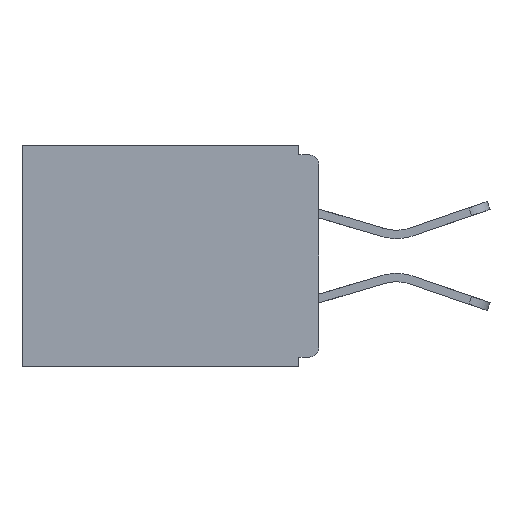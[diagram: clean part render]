
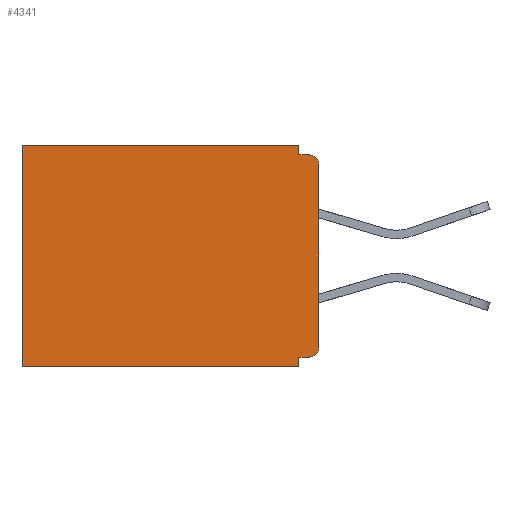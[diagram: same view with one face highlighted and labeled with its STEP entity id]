
A CAD part, left-side view. The second image highlights one B-rep face of the part: STEP entity #4341.
In plain terms, the highlighted planar face has unit normal (-1, 0, 0).
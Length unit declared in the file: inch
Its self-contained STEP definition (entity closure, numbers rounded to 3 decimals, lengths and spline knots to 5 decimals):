
#264 = VECTOR ( 'NONE', #6462, 39.37008 ) ;
#429 = LINE ( 'NONE', #3841, #842 ) ;
#657 = VECTOR ( 'NONE', #9580, 39.37008 ) ;
#702 = VECTOR ( 'NONE', #5959, 39.37008 ) ;
#765 = EDGE_CURVE ( 'NONE', #10484, #6599, #7056, .T. ) ;
#837 = EDGE_CURVE ( 'NONE', #10484, #2158, #3985, .T. ) ;
#842 = VECTOR ( 'NONE', #13046, 39.37008 ) ;
#1047 = CARTESIAN_POINT ( 'NONE',  ( 0.298, 0., -0.03 ) ) ;
#1114 = LINE ( 'NONE', #1964, #702 ) ;
#1277 = VERTEX_POINT ( 'NONE', #11123 ) ;
#1627 = EDGE_CURVE ( 'NONE', #6599, #11032, #429, .T. ) ;
#1770 = EDGE_LOOP ( 'NONE', ( #12987, #15090, #11916, #7099, #12322, #15769, #7024, #5704, #8337, #3221 ) ) ;
#1964 = CARTESIAN_POINT ( 'NONE',  ( 0.298, 0., 0. ) ) ;
#2158 = VERTEX_POINT ( 'NONE', #2825 ) ;
#2263 = DIRECTION ( 'NONE',  ( -1., 0., 0. ) ) ;
#2493 = CARTESIAN_POINT ( 'NONE',  ( 0.298, 0., -0.343 ) ) ;
#2712 = LINE ( 'NONE', #16042, #12008 ) ;
#2825 = CARTESIAN_POINT ( 'NONE',  ( 0.298, 0., -0.313 ) ) ;
#3004 = EDGE_CURVE ( 'NONE', #9972, #15395, #13359, .T. ) ;
#3078 = LINE ( 'NONE', #15502, #10525 ) ;
#3161 = CARTESIAN_POINT ( 'NONE',  ( 0.298, 0., -0.015 ) ) ;
#3221 = ORIENTED_EDGE ( 'NONE', *, *, #5200, .F. ) ;
#3610 = CARTESIAN_POINT ( 'NONE',  ( 0.298, 0.015, -0.328 ) ) ;
#3698 = DIRECTION ( 'NONE',  ( -1., 0., 0. ) ) ;
#3841 = CARTESIAN_POINT ( 'NONE',  ( 0.298, 0.031, -0.343 ) ) ;
#3985 = CIRCLE ( 'NONE', #14149, 0.015 ) ;
#4000 = DIRECTION ( 'NONE',  ( 0., 0., -1. ) ) ;
#4341 = ADVANCED_FACE ( 'NONE', ( #10231 ), #12079, .F. ) ;
#4699 = DIRECTION ( 'NONE',  ( 0., 1., 0. ) ) ;
#4863 = AXIS2_PLACEMENT_3D ( 'NONE', #5848, #9821, #5898 ) ;
#5200 = EDGE_CURVE ( 'NONE', #9972, #2158, #1114, .T. ) ;
#5704 = ORIENTED_EDGE ( 'NONE', *, *, #765, .F. ) ;
#5848 = CARTESIAN_POINT ( 'NONE',  ( 0.298, 0., 0. ) ) ;
#5898 = DIRECTION ( 'NONE',  ( 0., 0., -1. ) ) ;
#5959 = DIRECTION ( 'NONE',  ( 0., 0., -1. ) ) ;
#6462 = DIRECTION ( 'NONE',  ( 0., 1., 0. ) ) ;
#6599 = VERTEX_POINT ( 'NONE', #15489 ) ;
#6679 = CARTESIAN_POINT ( 'NONE',  ( 0.298, 0.46, -0.343 ) ) ;
#6841 = CARTESIAN_POINT ( 'NONE',  ( 0.298, 0.031, -0.343 ) ) ;
#7024 = ORIENTED_EDGE ( 'NONE', *, *, #1627, .F. ) ;
#7031 = CARTESIAN_POINT ( 'NONE',  ( 0.298, 0.015, -0.313 ) ) ;
#7056 = LINE ( 'NONE', #8431, #11416 ) ;
#7099 = ORIENTED_EDGE ( 'NONE', *, *, #9230, .T. ) ;
#7372 = DIRECTION ( 'NONE',  ( 0., 1., 0. ) ) ;
#7531 = CARTESIAN_POINT ( 'NONE',  ( 0.298, 0.015, -0.03 ) ) ;
#8220 = VERTEX_POINT ( 'NONE', #12640 ) ;
#8337 = ORIENTED_EDGE ( 'NONE', *, *, #837, .T. ) ;
#8431 = CARTESIAN_POINT ( 'NONE',  ( 0.298, 0., -0.328 ) ) ;
#8561 = LINE ( 'NONE', #13808, #15483 ) ;
#9230 = EDGE_CURVE ( 'NONE', #13248, #1277, #8561, .T. ) ;
#9345 = LINE ( 'NONE', #3161, #657 ) ;
#9447 = CARTESIAN_POINT ( 'NONE',  ( 0.298, 0.031, 0. ) ) ;
#9554 = LINE ( 'NONE', #2493, #264 ) ;
#9580 = DIRECTION ( 'NONE',  ( 0., -1., 0. ) ) ;
#9821 = DIRECTION ( 'NONE',  ( 1., 0., 0. ) ) ;
#9972 = VERTEX_POINT ( 'NONE', #1047 ) ;
#10231 = FACE_OUTER_BOUND ( 'NONE', #1770, .T. ) ;
#10484 = VERTEX_POINT ( 'NONE', #3610 ) ;
#10525 = VECTOR ( 'NONE', #16702, 39.37008 ) ;
#10628 = EDGE_CURVE ( 'NONE', #1277, #12233, #2712, .T. ) ;
#11032 = VERTEX_POINT ( 'NONE', #6841 ) ;
#11123 = CARTESIAN_POINT ( 'NONE',  ( 0.298, 0.46, 0. ) ) ;
#11416 = VECTOR ( 'NONE', #4699, 39.37008 ) ;
#11916 = ORIENTED_EDGE ( 'NONE', *, *, #16819, .F. ) ;
#12008 = VECTOR ( 'NONE', #15984, 39.37008 ) ;
#12079 = PLANE ( 'NONE',  #4863 ) ;
#12233 = VERTEX_POINT ( 'NONE', #6679 ) ;
#12322 = ORIENTED_EDGE ( 'NONE', *, *, #10628, .T. ) ;
#12640 = CARTESIAN_POINT ( 'NONE',  ( 0.298, 0.031, -0.015 ) ) ;
#12987 = ORIENTED_EDGE ( 'NONE', *, *, #3004, .T. ) ;
#13046 = DIRECTION ( 'NONE',  ( 0., 0., -1. ) ) ;
#13248 = VERTEX_POINT ( 'NONE', #9447 ) ;
#13359 = CIRCLE ( 'NONE', #14079, 0.015 ) ;
#13808 = CARTESIAN_POINT ( 'NONE',  ( 0.298, 0., 0. ) ) ;
#14023 = EDGE_CURVE ( 'NONE', #8220, #15395, #9345, .T. ) ;
#14079 = AXIS2_PLACEMENT_3D ( 'NONE', #7531, #2263, #16785 ) ;
#14149 = AXIS2_PLACEMENT_3D ( 'NONE', #7031, #3698, #4000 ) ;
#14386 = EDGE_CURVE ( 'NONE', #11032, #12233, #9554, .T. ) ;
#14854 = CARTESIAN_POINT ( 'NONE',  ( 0.298, 0.015, -0.015 ) ) ;
#15090 = ORIENTED_EDGE ( 'NONE', *, *, #14023, .F. ) ;
#15395 = VERTEX_POINT ( 'NONE', #14854 ) ;
#15483 = VECTOR ( 'NONE', #7372, 39.37008 ) ;
#15489 = CARTESIAN_POINT ( 'NONE',  ( 0.298, 0.031, -0.328 ) ) ;
#15502 = CARTESIAN_POINT ( 'NONE',  ( 0.298, 0.031, -0.343 ) ) ;
#15769 = ORIENTED_EDGE ( 'NONE', *, *, #14386, .F. ) ;
#15984 = DIRECTION ( 'NONE',  ( 0., 0., -1. ) ) ;
#16042 = CARTESIAN_POINT ( 'NONE',  ( 0.298, 0.46, 0. ) ) ;
#16702 = DIRECTION ( 'NONE',  ( 0., 0., -1. ) ) ;
#16785 = DIRECTION ( 'NONE',  ( 0., 0., -1. ) ) ;
#16819 = EDGE_CURVE ( 'NONE', #13248, #8220, #3078, .T. ) ;
